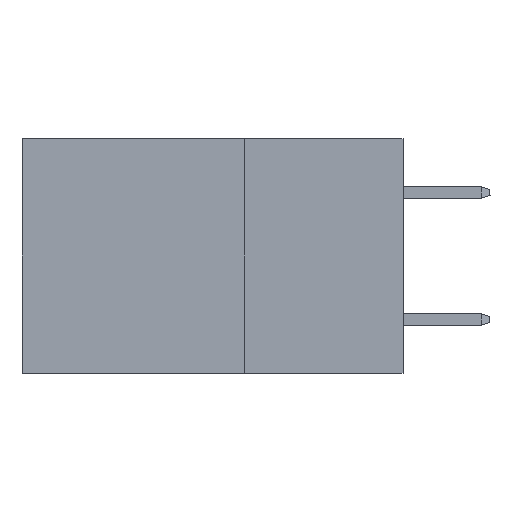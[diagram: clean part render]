
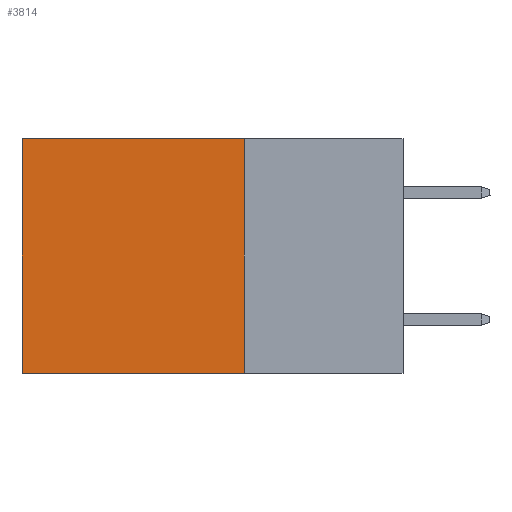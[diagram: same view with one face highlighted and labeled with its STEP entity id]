
A CAD part, left-side view. The second image highlights one B-rep face of the part: STEP entity #3814.
In plain terms, the highlighted planar face has unit normal (-1, 0, 0).
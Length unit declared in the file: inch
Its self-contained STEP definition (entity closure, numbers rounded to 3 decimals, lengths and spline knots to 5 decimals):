
#612 = EDGE_CURVE ( 'NONE', #26162, #4300, #26545, .T. ) ;
#3010 = EDGE_CURVE ( 'NONE', #4300, #15680, #29267, .T. ) ;
#3814 = ADVANCED_FACE ( 'NONE', ( #17722 ), #14925, .F. ) ;
#4300 = VERTEX_POINT ( 'NONE', #24237 ) ;
#8402 = DIRECTION ( 'NONE',  ( 0., 0., -1. ) ) ;
#9809 = ORIENTED_EDGE ( 'NONE', *, *, #3010, .F. ) ;
#11180 = CARTESIAN_POINT ( 'NONE',  ( 0.2875, 0.6, 0. ) ) ;
#11260 = VECTOR ( 'NONE', #12779, 39.37008 ) ;
#12779 = DIRECTION ( 'NONE',  ( 0., 0., -1. ) ) ;
#14486 = LINE ( 'NONE', #14837, #24207 ) ;
#14837 = CARTESIAN_POINT ( 'NONE',  ( 0.2875, 0.25, 0. ) ) ;
#14925 = PLANE ( 'NONE',  #26974 ) ;
#15090 = CARTESIAN_POINT ( 'NONE',  ( 0.2875, 0.25, 0. ) ) ;
#15680 = VERTEX_POINT ( 'NONE', #26988 ) ;
#16099 = CARTESIAN_POINT ( 'NONE',  ( 0.2875, 0.25, 0. ) ) ;
#16564 = CARTESIAN_POINT ( 'NONE',  ( 0.2875, 0.25, -0.37 ) ) ;
#16643 = ORIENTED_EDGE ( 'NONE', *, *, #30460, .T. ) ;
#16682 = EDGE_CURVE ( 'NONE', #17441, #15680, #19391, .T. ) ;
#17441 = VERTEX_POINT ( 'NONE', #29208 ) ;
#17722 = FACE_OUTER_BOUND ( 'NONE', #23718, .T. ) ;
#19391 = LINE ( 'NONE', #11180, #21996 ) ;
#20444 = CARTESIAN_POINT ( 'NONE',  ( 0.2875, 0.25, 0. ) ) ;
#20836 = VECTOR ( 'NONE', #31859, 39.37008 ) ;
#21996 = VECTOR ( 'NONE', #8402, 39.37008 ) ;
#23718 = EDGE_LOOP ( 'NONE', ( #24423, #9809, #31502, #16643 ) ) ;
#24207 = VECTOR ( 'NONE', #33278, 39.37008 ) ;
#24237 = CARTESIAN_POINT ( 'NONE',  ( 0.2875, 0.25, -0.37 ) ) ;
#24423 = ORIENTED_EDGE ( 'NONE', *, *, #16682, .T. ) ;
#25718 = DIRECTION ( 'NONE',  ( 1., 0., 0. ) ) ;
#26162 = VERTEX_POINT ( 'NONE', #20444 ) ;
#26545 = LINE ( 'NONE', #16099, #11260 ) ;
#26974 = AXIS2_PLACEMENT_3D ( 'NONE', #15090, #25718, #33705 ) ;
#26988 = CARTESIAN_POINT ( 'NONE',  ( 0.2875, 0.6, -0.37 ) ) ;
#29208 = CARTESIAN_POINT ( 'NONE',  ( 0.2875, 0.6, 0. ) ) ;
#29267 = LINE ( 'NONE', #16564, #20836 ) ;
#30460 = EDGE_CURVE ( 'NONE', #26162, #17441, #14486, .T. ) ;
#31502 = ORIENTED_EDGE ( 'NONE', *, *, #612, .F. ) ;
#31859 = DIRECTION ( 'NONE',  ( 0., 1., 0. ) ) ;
#33278 = DIRECTION ( 'NONE',  ( 0., 1., 0. ) ) ;
#33705 = DIRECTION ( 'NONE',  ( 0., 0., -1. ) ) ;
